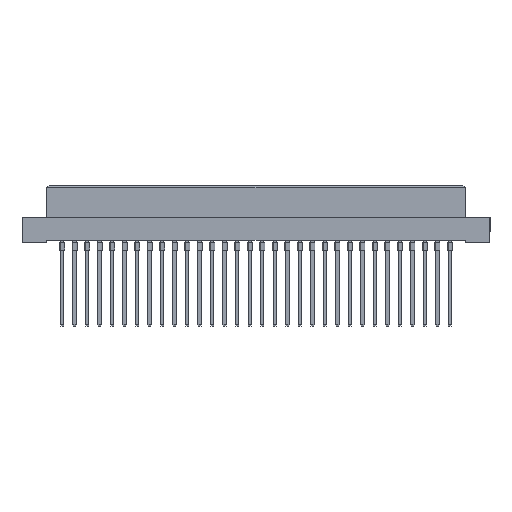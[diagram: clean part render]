
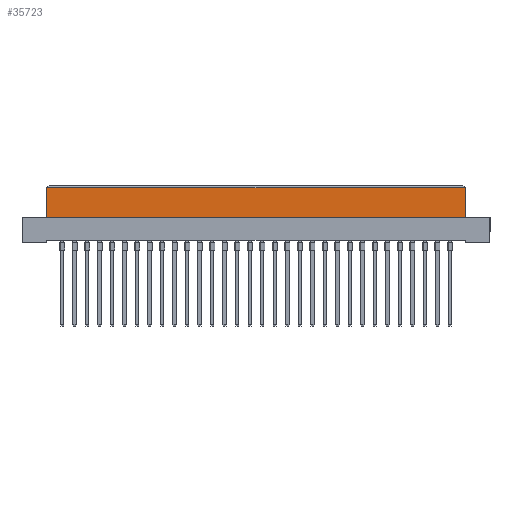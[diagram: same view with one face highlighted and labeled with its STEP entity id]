
A CAD part, top view. The second image highlights one B-rep face of the part: STEP entity #35723.
In plain terms, the highlighted planar face has unit normal (0, 0, 1).
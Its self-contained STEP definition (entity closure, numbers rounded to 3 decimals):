
#180 = EDGE_LOOP ( 'NONE', ( #22937, #24212, #29451, #29266 ) ) ;
#1954 = EDGE_CURVE ( 'NONE', #40760, #15221, #29948, .T. ) ;
#3840 = CARTESIAN_POINT ( 'NONE',  ( -42.5, -0.5, 4.25 ) ) ;
#4530 = EDGE_CURVE ( 'NONE', #13798, #36607, #20067, .T. ) ;
#4824 = DIRECTION ( 'NONE',  ( 0., 0., 1. ) ) ;
#5214 = CARTESIAN_POINT ( 'NONE',  ( -42.5, -0.5, 4.25 ) ) ;
#6834 = VECTOR ( 'NONE', #38627, 1000. ) ;
#7099 = CARTESIAN_POINT ( 'NONE',  ( 42.5, -6.4, 4.25 ) ) ;
#7448 = EDGE_CURVE ( 'NONE', #40760, #13798, #31991, .T. ) ;
#7731 = CARTESIAN_POINT ( 'NONE',  ( 42.5, -6.4, 4.25 ) ) ;
#8406 = CARTESIAN_POINT ( 'NONE',  ( 42.5, -0.5, 4.25 ) ) ;
#10094 = CARTESIAN_POINT ( 'NONE',  ( 42.5, -6.4, 4.25 ) ) ;
#10440 = DIRECTION ( 'NONE',  ( 0., 1., 0. ) ) ;
#10629 = DIRECTION ( 'NONE',  ( -1., 0., 0. ) ) ;
#13798 = VERTEX_POINT ( 'NONE', #7099 ) ;
#15221 = VERTEX_POINT ( 'NONE', #3840 ) ;
#17472 = LINE ( 'NONE', #5214, #25075 ) ;
#19030 = EDGE_CURVE ( 'NONE', #36607, #15221, #17472, .T. ) ;
#19946 = CARTESIAN_POINT ( 'NONE',  ( 42.5, -6.4, 4.25 ) ) ;
#20067 = LINE ( 'NONE', #10094, #23555 ) ;
#20627 = PLANE ( 'NONE',  #30206 ) ;
#22937 = ORIENTED_EDGE ( 'NONE', *, *, #4530, .T. ) ;
#23555 = VECTOR ( 'NONE', #32525, 1000. ) ;
#24212 = ORIENTED_EDGE ( 'NONE', *, *, #19030, .T. ) ;
#24269 = CARTESIAN_POINT ( 'NONE',  ( -42.5, -6.4, 4.25 ) ) ;
#25075 = VECTOR ( 'NONE', #10629, 1000. ) ;
#29266 = ORIENTED_EDGE ( 'NONE', *, *, #7448, .T. ) ;
#29451 = ORIENTED_EDGE ( 'NONE', *, *, #1954, .F. ) ;
#29948 = LINE ( 'NONE', #39490, #32742 ) ;
#30206 = AXIS2_PLACEMENT_3D ( 'NONE', #7731, #4824, #33286 ) ;
#31991 = LINE ( 'NONE', #19946, #6834 ) ;
#32525 = DIRECTION ( 'NONE',  ( 0., 1., 0. ) ) ;
#32742 = VECTOR ( 'NONE', #10440, 1000. ) ;
#33286 = DIRECTION ( 'NONE',  ( 1., 0., 0. ) ) ;
#35723 = ADVANCED_FACE ( 'NONE', ( #40675 ), #20627, .T. ) ;
#36607 = VERTEX_POINT ( 'NONE', #8406 ) ;
#38627 = DIRECTION ( 'NONE',  ( 1., 0., 0. ) ) ;
#39490 = CARTESIAN_POINT ( 'NONE',  ( -42.5, -6.4, 4.25 ) ) ;
#40675 = FACE_OUTER_BOUND ( 'NONE', #180, .T. ) ;
#40760 = VERTEX_POINT ( 'NONE', #24269 ) ;
